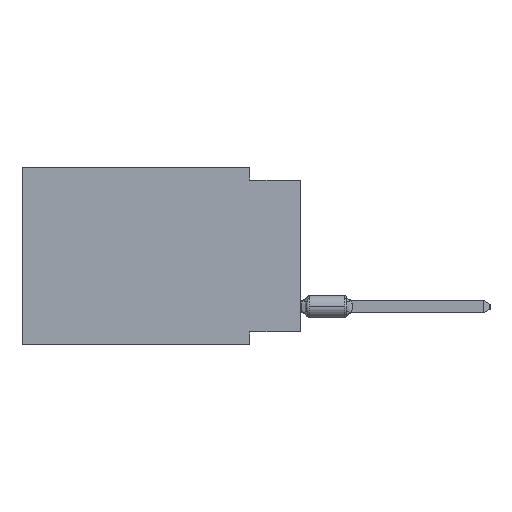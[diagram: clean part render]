
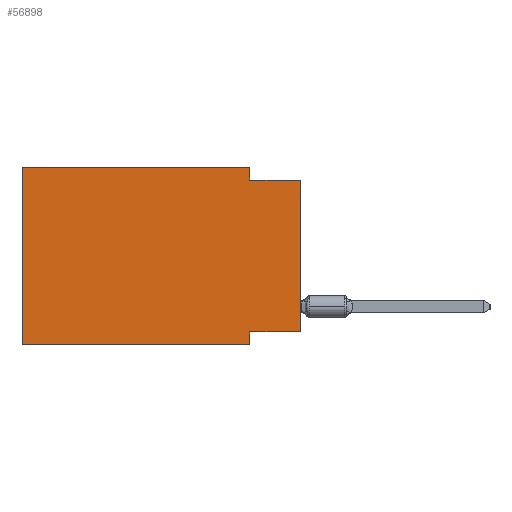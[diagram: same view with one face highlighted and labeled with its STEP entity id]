
A CAD part, left-side view. The second image highlights one B-rep face of the part: STEP entity #56898.
In plain terms, the highlighted planar face has unit normal (-1, 0, 0).
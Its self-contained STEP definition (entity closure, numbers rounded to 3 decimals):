
#277 = DIRECTION ( 'NONE',  ( 0., 0., 1. ) ) ;
#645 = VECTOR ( 'NONE', #40586, 1000. ) ;
#739 = VERTEX_POINT ( 'NONE', #34035 ) ;
#1347 = ORIENTED_EDGE ( 'NONE', *, *, #47217, .F. ) ;
#4685 = CARTESIAN_POINT ( 'NONE',  ( 0., 13.97, -8.89 ) ) ;
#5351 = EDGE_CURVE ( 'NONE', #34070, #32919, #65808, .T. ) ;
#7608 = ORIENTED_EDGE ( 'NONE', *, *, #37170, .F. ) ;
#8053 = CARTESIAN_POINT ( 'NONE',  ( 0., 13.97, 0. ) ) ;
#10628 = EDGE_CURVE ( 'NONE', #52052, #47858, #43788, .T. ) ;
#12731 = ORIENTED_EDGE ( 'NONE', *, *, #32074, .T. ) ;
#13420 = ORIENTED_EDGE ( 'NONE', *, *, #31736, .F. ) ;
#15885 = LINE ( 'NONE', #37679, #33242 ) ;
#16453 = DIRECTION ( 'NONE',  ( 0., -1., 0. ) ) ;
#16656 = VECTOR ( 'NONE', #33658, 1000. ) ;
#17301 = CARTESIAN_POINT ( 'NONE',  ( 0., 13.97, 0. ) ) ;
#18809 = LINE ( 'NONE', #19840, #32283 ) ;
#19523 = VECTOR ( 'NONE', #48462, 1000. ) ;
#19840 = CARTESIAN_POINT ( 'NONE',  ( 0., 2.54, 0. ) ) ;
#20672 = VERTEX_POINT ( 'NONE', #53072 ) ;
#21519 = VECTOR ( 'NONE', #277, 1000. ) ;
#26057 = VECTOR ( 'NONE', #16453, 1000. ) ;
#26145 = AXIS2_PLACEMENT_3D ( 'NONE', #55861, #45467, #50849 ) ;
#27520 = CARTESIAN_POINT ( 'NONE',  ( 0., 13.97, 0. ) ) ;
#28341 = FACE_OUTER_BOUND ( 'NONE', #36800, .T. ) ;
#31736 = EDGE_CURVE ( 'NONE', #33938, #34029, #43605, .T. ) ;
#31795 = CARTESIAN_POINT ( 'NONE',  ( 0., 2.54, -0.635 ) ) ;
#32074 = EDGE_CURVE ( 'NONE', #20672, #47858, #59945, .T. ) ;
#32283 = VECTOR ( 'NONE', #46650, 1000. ) ;
#32331 = ORIENTED_EDGE ( 'NONE', *, *, #42280, .F. ) ;
#32919 = VERTEX_POINT ( 'NONE', #62242 ) ;
#33242 = VECTOR ( 'NONE', #59475, 1000. ) ;
#33417 = CARTESIAN_POINT ( 'NONE',  ( 0., 0., -0.635 ) ) ;
#33658 = DIRECTION ( 'NONE',  ( 0., -1., 0. ) ) ;
#33938 = VERTEX_POINT ( 'NONE', #17301 ) ;
#34029 = VERTEX_POINT ( 'NONE', #40115 ) ;
#34035 = CARTESIAN_POINT ( 'NONE',  ( 0., 2.54, -8.255 ) ) ;
#34049 = PLANE ( 'NONE',  #26145 ) ;
#34070 = VERTEX_POINT ( 'NONE', #4685 ) ;
#35783 = EDGE_CURVE ( 'NONE', #34070, #33938, #62718, .T. ) ;
#36506 = CARTESIAN_POINT ( 'NONE',  ( 0., 2.54, -8.89 ) ) ;
#36800 = EDGE_LOOP ( 'NONE', ( #12731, #37245, #1347, #13420, #69190, #66672, #7608, #32331 ) ) ;
#37170 = EDGE_CURVE ( 'NONE', #739, #32919, #63661, .T. ) ;
#37245 = ORIENTED_EDGE ( 'NONE', *, *, #10628, .F. ) ;
#37679 = CARTESIAN_POINT ( 'NONE',  ( 0., 0., -8.255 ) ) ;
#39703 = CARTESIAN_POINT ( 'NONE',  ( 0., 0., -0.635 ) ) ;
#40115 = CARTESIAN_POINT ( 'NONE',  ( 0., 2.54, 0. ) ) ;
#40586 = DIRECTION ( 'NONE',  ( 0., 0., 1. ) ) ;
#42280 = EDGE_CURVE ( 'NONE', #20672, #739, #15885, .T. ) ;
#43605 = LINE ( 'NONE', #27520, #26057 ) ;
#43788 = LINE ( 'NONE', #33417, #19523 ) ;
#44590 = CARTESIAN_POINT ( 'NONE',  ( 0., 0., 0. ) ) ;
#45467 = DIRECTION ( 'NONE',  ( 1., 0., 0. ) ) ;
#46650 = DIRECTION ( 'NONE',  ( 0., 0., -1. ) ) ;
#47217 = EDGE_CURVE ( 'NONE', #34029, #52052, #18809, .T. ) ;
#47858 = VERTEX_POINT ( 'NONE', #39703 ) ;
#48462 = DIRECTION ( 'NONE',  ( 0., -1., 0. ) ) ;
#50849 = DIRECTION ( 'NONE',  ( 0., 0., -1. ) ) ;
#52052 = VERTEX_POINT ( 'NONE', #31795 ) ;
#53072 = CARTESIAN_POINT ( 'NONE',  ( 0., 0., -8.255 ) ) ;
#55861 = CARTESIAN_POINT ( 'NONE',  ( 0., 13.97, 0. ) ) ;
#56898 = ADVANCED_FACE ( 'NONE', ( #28341 ), #34049, .F. ) ;
#58312 = DIRECTION ( 'NONE',  ( 0., 0., -1. ) ) ;
#58982 = VECTOR ( 'NONE', #58312, 1000. ) ;
#59475 = DIRECTION ( 'NONE',  ( 0., 1., 0. ) ) ;
#59945 = LINE ( 'NONE', #44590, #21519 ) ;
#62242 = CARTESIAN_POINT ( 'NONE',  ( 0., 2.54, -8.89 ) ) ;
#62718 = LINE ( 'NONE', #8053, #645 ) ;
#63661 = LINE ( 'NONE', #36506, #58982 ) ;
#65808 = LINE ( 'NONE', #66510, #16656 ) ;
#66510 = CARTESIAN_POINT ( 'NONE',  ( 0., 13.97, -8.89 ) ) ;
#66672 = ORIENTED_EDGE ( 'NONE', *, *, #5351, .T. ) ;
#69190 = ORIENTED_EDGE ( 'NONE', *, *, #35783, .F. ) ;
